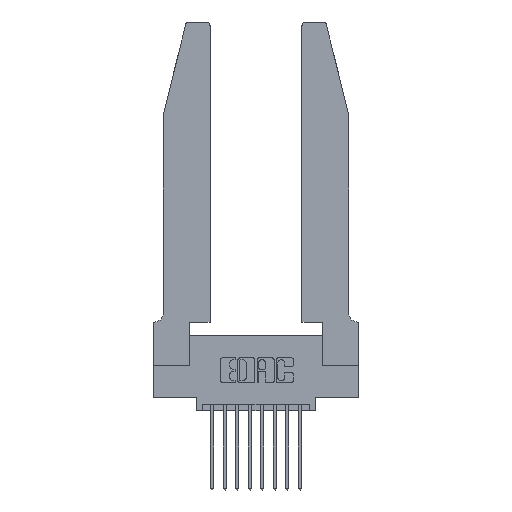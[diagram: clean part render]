
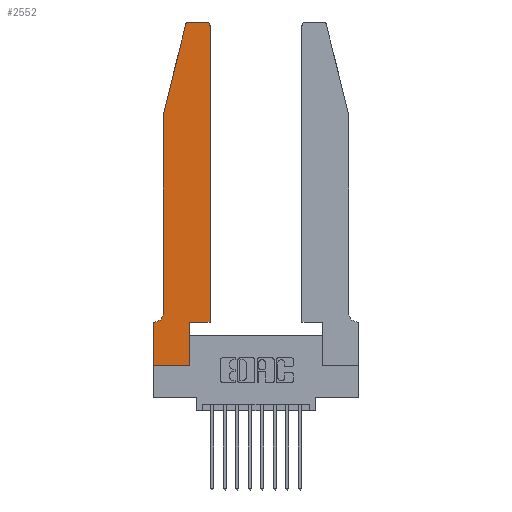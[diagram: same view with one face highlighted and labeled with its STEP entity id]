
A CAD part, top view. The second image highlights one B-rep face of the part: STEP entity #2552.
In plain terms, the highlighted planar face has unit normal (0, 0, 1).
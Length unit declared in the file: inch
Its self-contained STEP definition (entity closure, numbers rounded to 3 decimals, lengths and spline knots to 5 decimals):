
#111 = DIRECTION ( 'NONE',  ( 1., 0., 0. ) ) ;
#236 = CARTESIAN_POINT ( 'NONE',  ( 0.2865, 0., 0.37 ) ) ;
#684 = VERTEX_POINT ( 'NONE', #6020 ) ;
#917 = VECTOR ( 'NONE', #14908, 39.37008 ) ;
#1110 = VERTEX_POINT ( 'NONE', #14769 ) ;
#1312 = EDGE_CURVE ( 'NONE', #7245, #15757, #12235, .T. ) ;
#1328 = LINE ( 'NONE', #2805, #10788 ) ;
#1338 = EDGE_CURVE ( 'NONE', #1387, #12772, #2548, .T. ) ;
#1386 = ORIENTED_EDGE ( 'NONE', *, *, #2128, .T. ) ;
#1387 = VERTEX_POINT ( 'NONE', #8181 ) ;
#1474 = AXIS2_PLACEMENT_3D ( 'NONE', #8495, #7723, #7625 ) ;
#1651 = AXIS2_PLACEMENT_3D ( 'NONE', #11901, #13591, #12595 ) ;
#1867 = EDGE_CURVE ( 'NONE', #15757, #7047, #2535, .T. ) ;
#1902 = LINE ( 'NONE', #5193, #14035 ) ;
#1965 = CARTESIAN_POINT ( 'NONE',  ( 0.2865, 0.35, 0.37 ) ) ;
#2128 = EDGE_CURVE ( 'NONE', #684, #1110, #11311, .T. ) ;
#2338 = AXIS2_PLACEMENT_3D ( 'NONE', #14733, #7675, #111 ) ;
#2535 = CIRCLE ( 'NONE', #12020, 0.03 ) ;
#2548 = CIRCLE ( 'NONE', #1651, 0.07 ) ;
#2552 = ADVANCED_FACE ( 'NONE', ( #3543 ), #7489, .T. ) ;
#2805 = CARTESIAN_POINT ( 'NONE',  ( 0.0755, 2., 0.37 ) ) ;
#2934 = LINE ( 'NONE', #1965, #11851 ) ;
#2937 = EDGE_LOOP ( 'NONE', ( #6737, #11631, #5255, #15633, #7120, #10700, #8875, #6050, #7920, #8482, #1386, #5518 ) ) ;
#3094 = CARTESIAN_POINT ( 'NONE',  ( 0.0755, 2., 0.37 ) ) ;
#3203 = CARTESIAN_POINT ( 'NONE',  ( 0.4505, 0.35, 0.37 ) ) ;
#3293 = DIRECTION ( 'NONE',  ( 0., 1., 0. ) ) ;
#3397 = CARTESIAN_POINT ( 'NONE',  ( 0.0755, 0.35, 0.37 ) ) ;
#3543 = FACE_OUTER_BOUND ( 'NONE', #2937, .T. ) ;
#3743 = CARTESIAN_POINT ( 'NONE',  ( 0., 0., 0.37 ) ) ;
#4255 = CIRCLE ( 'NONE', #2338, 0.03 ) ;
#4371 = DIRECTION ( 'NONE',  ( 1., 0., 0. ) ) ;
#4626 = EDGE_CURVE ( 'NONE', #10195, #7321, #9423, .T. ) ;
#4944 = VECTOR ( 'NONE', #8235, 39.37008 ) ;
#5193 = CARTESIAN_POINT ( 'NONE',  ( 0.0755, 2., 0.37 ) ) ;
#5255 = ORIENTED_EDGE ( 'NONE', *, *, #9725, .T. ) ;
#5393 = EDGE_CURVE ( 'NONE', #12772, #8641, #11226, .T. ) ;
#5410 = CARTESIAN_POINT ( 'NONE',  ( 0., 0., 0.37 ) ) ;
#5518 = ORIENTED_EDGE ( 'NONE', *, *, #14689, .T. ) ;
#5536 = LINE ( 'NONE', #5410, #917 ) ;
#5721 = CARTESIAN_POINT ( 'NONE',  ( 0.4505, 0.35, 0.37 ) ) ;
#5796 = CARTESIAN_POINT ( 'NONE',  ( 0.25487, 2.72718, 0.37 ) ) ;
#5924 = VECTOR ( 'NONE', #11865, 39.37008 ) ;
#6020 = CARTESIAN_POINT ( 'NONE',  ( 0.4505, 0.35, 0.37 ) ) ;
#6050 = ORIENTED_EDGE ( 'NONE', *, *, #4626, .T. ) ;
#6315 = CARTESIAN_POINT ( 'NONE',  ( 0.4205, 2.75, 0.37 ) ) ;
#6618 = DIRECTION ( 'NONE',  ( 1., 0., 0. ) ) ;
#6737 = ORIENTED_EDGE ( 'NONE', *, *, #1312, .T. ) ;
#7047 = VERTEX_POINT ( 'NONE', #5796 ) ;
#7120 = ORIENTED_EDGE ( 'NONE', *, *, #1338, .T. ) ;
#7245 = VERTEX_POINT ( 'NONE', #6315 ) ;
#7321 = VERTEX_POINT ( 'NONE', #236 ) ;
#7489 = PLANE ( 'NONE',  #1474 ) ;
#7625 = DIRECTION ( 'NONE',  ( 1., 0., 0. ) ) ;
#7675 = DIRECTION ( 'NONE',  ( 0., 0., 1. ) ) ;
#7723 = DIRECTION ( 'NONE',  ( 0., 0., 1. ) ) ;
#7920 = ORIENTED_EDGE ( 'NONE', *, *, #11711, .T. ) ;
#8120 = DIRECTION ( 'NONE',  ( 0., 0., 1. ) ) ;
#8181 = CARTESIAN_POINT ( 'NONE',  ( 0.0755, 0.42, 0.37 ) ) ;
#8235 = DIRECTION ( 'NONE',  ( 0., 1., 0. ) ) ;
#8482 = ORIENTED_EDGE ( 'NONE', *, *, #11014, .T. ) ;
#8495 = CARTESIAN_POINT ( 'NONE',  ( 0., 0.35, 0.37 ) ) ;
#8552 = LINE ( 'NONE', #3203, #14813 ) ;
#8563 = CARTESIAN_POINT ( 'NONE',  ( 0.2865, 0.35, 0.37 ) ) ;
#8641 = VERTEX_POINT ( 'NONE', #10568 ) ;
#8875 = ORIENTED_EDGE ( 'NONE', *, *, #10863, .T. ) ;
#9001 = DIRECTION ( 'NONE',  ( 0., -1., 0. ) ) ;
#9423 = LINE ( 'NONE', #14897, #12507 ) ;
#9496 = DIRECTION ( 'NONE',  ( -1., 0., 0. ) ) ;
#9609 = VERTEX_POINT ( 'NONE', #8563 ) ;
#9725 = EDGE_CURVE ( 'NONE', #7047, #15541, #1902, .T. ) ;
#10195 = VERTEX_POINT ( 'NONE', #3743 ) ;
#10568 = CARTESIAN_POINT ( 'NONE',  ( 0., 0.35, 0.37 ) ) ;
#10700 = ORIENTED_EDGE ( 'NONE', *, *, #5393, .T. ) ;
#10788 = VECTOR ( 'NONE', #9001, 39.37008 ) ;
#10841 = EDGE_CURVE ( 'NONE', #15541, #1387, #1328, .T. ) ;
#10863 = EDGE_CURVE ( 'NONE', #8641, #10195, #5536, .T. ) ;
#11014 = EDGE_CURVE ( 'NONE', #9609, #684, #8552, .T. ) ;
#11138 = DIRECTION ( 'NONE',  ( -0.239, -0.971, 0. ) ) ;
#11226 = LINE ( 'NONE', #3397, #14332 ) ;
#11311 = LINE ( 'NONE', #5721, #4944 ) ;
#11410 = CARTESIAN_POINT ( 'NONE',  ( 0.0055, 0.35, 0.37 ) ) ;
#11631 = ORIENTED_EDGE ( 'NONE', *, *, #1867, .T. ) ;
#11711 = EDGE_CURVE ( 'NONE', #7321, #9609, #2934, .T. ) ;
#11755 = CARTESIAN_POINT ( 'NONE',  ( 0.284, 2.72, 0.37 ) ) ;
#11851 = VECTOR ( 'NONE', #3293, 39.37008 ) ;
#11865 = DIRECTION ( 'NONE',  ( -1., 0., 0. ) ) ;
#11901 = CARTESIAN_POINT ( 'NONE',  ( 0.0055, 0.42, 0.37 ) ) ;
#12020 = AXIS2_PLACEMENT_3D ( 'NONE', #11755, #8120, #4371 ) ;
#12235 = LINE ( 'NONE', #12631, #5924 ) ;
#12507 = VECTOR ( 'NONE', #6618, 39.37008 ) ;
#12595 = DIRECTION ( 'NONE',  ( -1., 0., 0. ) ) ;
#12631 = CARTESIAN_POINT ( 'NONE',  ( 0.2605, 2.75, 0.37 ) ) ;
#12772 = VERTEX_POINT ( 'NONE', #11410 ) ;
#12823 = DIRECTION ( 'NONE',  ( 1., 0., 0. ) ) ;
#13591 = DIRECTION ( 'NONE',  ( 0., 0., -1. ) ) ;
#14035 = VECTOR ( 'NONE', #11138, 39.37008 ) ;
#14268 = CARTESIAN_POINT ( 'NONE',  ( 0.284, 2.75, 0.37 ) ) ;
#14332 = VECTOR ( 'NONE', #9496, 39.37008 ) ;
#14689 = EDGE_CURVE ( 'NONE', #1110, #7245, #4255, .T. ) ;
#14733 = CARTESIAN_POINT ( 'NONE',  ( 0.4205, 2.72, 0.37 ) ) ;
#14769 = CARTESIAN_POINT ( 'NONE',  ( 0.4505, 2.72, 0.37 ) ) ;
#14813 = VECTOR ( 'NONE', #12823, 39.37008 ) ;
#14897 = CARTESIAN_POINT ( 'NONE',  ( 0., 0., 0.37 ) ) ;
#14908 = DIRECTION ( 'NONE',  ( 0., -1., 0. ) ) ;
#15541 = VERTEX_POINT ( 'NONE', #3094 ) ;
#15633 = ORIENTED_EDGE ( 'NONE', *, *, #10841, .T. ) ;
#15757 = VERTEX_POINT ( 'NONE', #14268 ) ;
